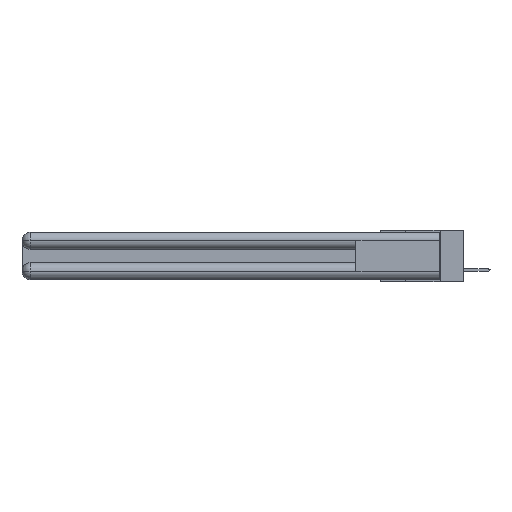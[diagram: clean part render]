
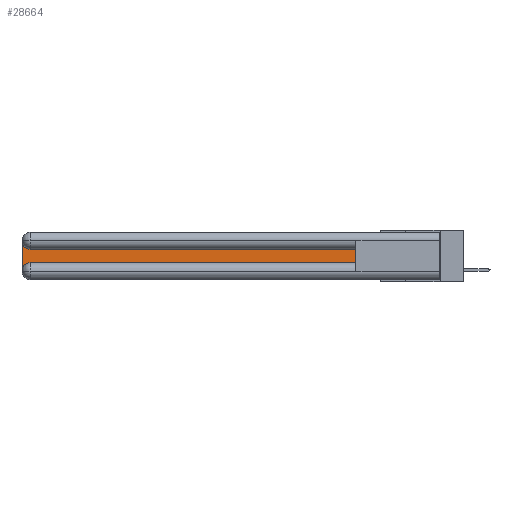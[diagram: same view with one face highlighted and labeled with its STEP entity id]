
A CAD part, left-side view. The second image highlights one B-rep face of the part: STEP entity #28664.
In plain terms, the highlighted planar face has unit normal (-1, 0, 0).
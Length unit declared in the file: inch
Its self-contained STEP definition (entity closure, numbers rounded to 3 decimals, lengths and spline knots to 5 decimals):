
#692 = ORIENTED_EDGE ( 'NONE', *, *, #6656, .T. ) ;
#758 = VERTEX_POINT ( 'NONE', #31665 ) ;
#2357 = VERTEX_POINT ( 'NONE', #27440 ) ;
#2681 = LINE ( 'NONE', #13148, #32057 ) ;
#3174 = EDGE_CURVE ( 'NONE', #2357, #21669, #13123, .T. ) ;
#3436 = VERTEX_POINT ( 'NONE', #14142 ) ;
#4015 = CARTESIAN_POINT ( 'NONE',  ( 0.075, 2.94, -0.2775 ) ) ;
#4381 = DIRECTION ( 'NONE',  ( 1., 0., 0. ) ) ;
#5553 = ORIENTED_EDGE ( 'NONE', *, *, #3174, .T. ) ;
#6656 = EDGE_CURVE ( 'NONE', #30968, #30759, #2681, .T. ) ;
#7702 = DIRECTION ( 'NONE',  ( 0., 0., -1. ) ) ;
#8260 = LINE ( 'NONE', #10298, #15357 ) ;
#8753 = ORIENTED_EDGE ( 'NONE', *, *, #13589, .T. ) ;
#8968 = CARTESIAN_POINT ( 'NONE',  ( 0.075, 0.6, -0.2175 ) ) ;
#9928 = CARTESIAN_POINT ( 'NONE',  ( 0.075, 3., -0.2175 ) ) ;
#10298 = CARTESIAN_POINT ( 'NONE',  ( 0.075, 0.6, -0.1225 ) ) ;
#12184 = ORIENTED_EDGE ( 'NONE', *, *, #13345, .T. ) ;
#12828 = AXIS2_PLACEMENT_3D ( 'NONE', #4015, #4381, #21111 ) ;
#12969 = DIRECTION ( 'NONE',  ( 0., 1., 0. ) ) ;
#13123 = LINE ( 'NONE', #9928, #26507 ) ;
#13148 = CARTESIAN_POINT ( 'NONE',  ( 0.075, 0.6, -0.2175 ) ) ;
#13345 = EDGE_CURVE ( 'NONE', #30759, #3436, #27361, .T. ) ;
#13589 = EDGE_CURVE ( 'NONE', #21669, #30968, #21053, .T. ) ;
#14142 = CARTESIAN_POINT ( 'NONE',  ( 0.075, 0.6, -0.1225 ) ) ;
#15357 = VECTOR ( 'NONE', #12969, 39.37008 ) ;
#15645 = CARTESIAN_POINT ( 'NONE',  ( 0.075, 2.94, -0.0625 ) ) ;
#17080 = EDGE_CURVE ( 'NONE', #3436, #758, #8260, .T. ) ;
#17138 = AXIS2_PLACEMENT_3D ( 'NONE', #15645, #23732, #7702 ) ;
#18198 = ORIENTED_EDGE ( 'NONE', *, *, #17080, .T. ) ;
#21053 = CIRCLE ( 'NONE', #12828, 0.06 ) ;
#21070 = CIRCLE ( 'NONE', #17138, 0.06 ) ;
#21111 = DIRECTION ( 'NONE',  ( 0., 0., -1. ) ) ;
#21176 = DIRECTION ( 'NONE',  ( 0., -1., 0. ) ) ;
#21669 = VERTEX_POINT ( 'NONE', #24425 ) ;
#22173 = PLANE ( 'NONE',  #25887 ) ;
#23642 = EDGE_LOOP ( 'NONE', ( #18198, #30534, #5553, #8753, #692, #12184 ) ) ;
#23732 = DIRECTION ( 'NONE',  ( 1., 0., 0. ) ) ;
#24273 = CARTESIAN_POINT ( 'NONE',  ( 0.075, 0.6, -0.2175 ) ) ;
#24425 = CARTESIAN_POINT ( 'NONE',  ( 0.075, 3., -0.2775 ) ) ;
#24553 = CARTESIAN_POINT ( 'NONE',  ( 0.075, 3., -0.1225 ) ) ;
#25887 = AXIS2_PLACEMENT_3D ( 'NONE', #24553, #27472, #26985 ) ;
#26507 = VECTOR ( 'NONE', #31321, 39.37008 ) ;
#26985 = DIRECTION ( 'NONE',  ( 0., 0., -1. ) ) ;
#27361 = LINE ( 'NONE', #8968, #30277 ) ;
#27440 = CARTESIAN_POINT ( 'NONE',  ( 0.075, 3., -0.0625 ) ) ;
#27472 = DIRECTION ( 'NONE',  ( 1., 0., 0. ) ) ;
#27669 = DIRECTION ( 'NONE',  ( 0., 0., 1. ) ) ;
#28352 = CARTESIAN_POINT ( 'NONE',  ( 0.075, 2.94, -0.2175 ) ) ;
#28664 = ADVANCED_FACE ( 'NONE', ( #33272 ), #22173, .F. ) ;
#29188 = EDGE_CURVE ( 'NONE', #758, #2357, #21070, .T. ) ;
#30277 = VECTOR ( 'NONE', #27669, 39.37008 ) ;
#30534 = ORIENTED_EDGE ( 'NONE', *, *, #29188, .T. ) ;
#30759 = VERTEX_POINT ( 'NONE', #24273 ) ;
#30968 = VERTEX_POINT ( 'NONE', #28352 ) ;
#31321 = DIRECTION ( 'NONE',  ( 0., 0., -1. ) ) ;
#31665 = CARTESIAN_POINT ( 'NONE',  ( 0.075, 2.94, -0.1225 ) ) ;
#32057 = VECTOR ( 'NONE', #21176, 39.37008 ) ;
#33272 = FACE_OUTER_BOUND ( 'NONE', #23642, .T. ) ;
